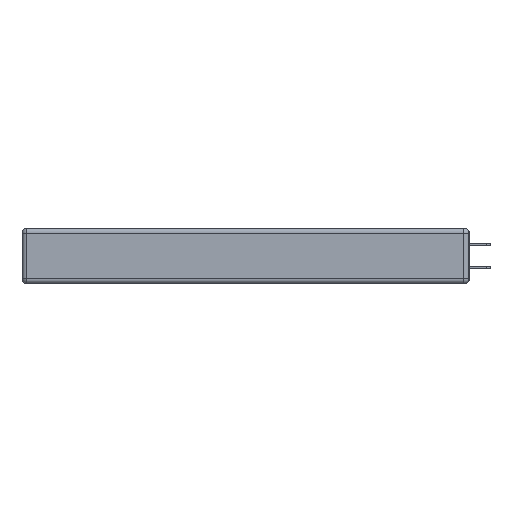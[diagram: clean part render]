
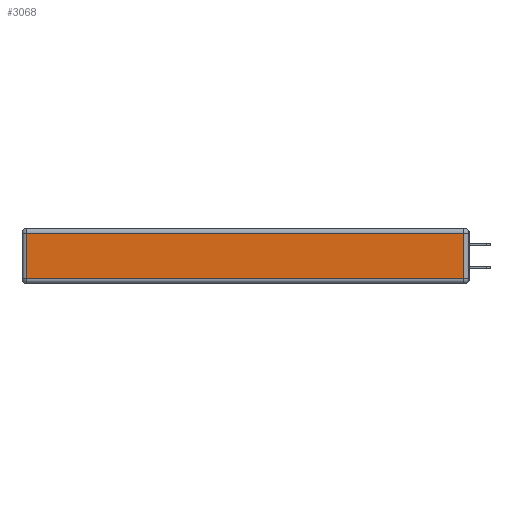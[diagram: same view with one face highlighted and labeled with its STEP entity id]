
A CAD part, left-side view. The second image highlights one B-rep face of the part: STEP entity #3068.
In plain terms, the highlighted planar face has unit normal (-1, 0, 0).
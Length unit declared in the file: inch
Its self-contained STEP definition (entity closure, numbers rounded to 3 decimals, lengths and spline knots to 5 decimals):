
#97 = CARTESIAN_POINT ( 'NONE',  ( 0., 2.72, -0.343 ) ) ;
#1035 = EDGE_CURVE ( 'NONE', #3423, #1359, #10766, .T. ) ;
#1359 = VERTEX_POINT ( 'NONE', #2898 ) ;
#1588 = CARTESIAN_POINT ( 'NONE',  ( 0., 0., -0.313 ) ) ;
#1816 = DIRECTION ( 'NONE',  ( 0., 0., 1. ) ) ;
#1874 = PLANE ( 'NONE',  #13687 ) ;
#2028 = ORIENTED_EDGE ( 'NONE', *, *, #1035, .T. ) ;
#2550 = FACE_OUTER_BOUND ( 'NONE', #21131, .T. ) ;
#2898 = CARTESIAN_POINT ( 'NONE',  ( 0., 0.03, -0.03 ) ) ;
#3068 = ADVANCED_FACE ( 'NONE', ( #2550 ), #1874, .T. ) ;
#3423 = VERTEX_POINT ( 'NONE', #15539 ) ;
#3523 = DIRECTION ( 'NONE',  ( 0., 0., -1. ) ) ;
#5363 = LINE ( 'NONE', #8226, #16827 ) ;
#6672 = ORIENTED_EDGE ( 'NONE', *, *, #12257, .T. ) ;
#6879 = DIRECTION ( 'NONE',  ( 0., -1., 0. ) ) ;
#7177 = ORIENTED_EDGE ( 'NONE', *, *, #19408, .T. ) ;
#8226 = CARTESIAN_POINT ( 'NONE',  ( 0., 2.75, -0.03 ) ) ;
#8332 = CARTESIAN_POINT ( 'NONE',  ( 0., 2.72, -0.03 ) ) ;
#9292 = EDGE_CURVE ( 'NONE', #10362, #3423, #16250, .T. ) ;
#9904 = CARTESIAN_POINT ( 'NONE',  ( 0., 2.72, -0.313 ) ) ;
#10362 = VERTEX_POINT ( 'NONE', #9904 ) ;
#10766 = LINE ( 'NONE', #20699, #14405 ) ;
#11316 = VECTOR ( 'NONE', #3523, 39.37008 ) ;
#11708 = DIRECTION ( 'NONE',  ( 0., 1., 0. ) ) ;
#12257 = EDGE_CURVE ( 'NONE', #20969, #10362, #16113, .T. ) ;
#12524 = DIRECTION ( 'NONE',  ( -1., 0., 0. ) ) ;
#13687 = AXIS2_PLACEMENT_3D ( 'NONE', #21454, #12524, #1816 ) ;
#14405 = VECTOR ( 'NONE', #22496, 39.37008 ) ;
#15539 = CARTESIAN_POINT ( 'NONE',  ( 0., 0.03, -0.313 ) ) ;
#16113 = LINE ( 'NONE', #97, #11316 ) ;
#16250 = LINE ( 'NONE', #1588, #20176 ) ;
#16827 = VECTOR ( 'NONE', #11708, 39.37008 ) ;
#19408 = EDGE_CURVE ( 'NONE', #1359, #20969, #5363, .T. ) ;
#20176 = VECTOR ( 'NONE', #6879, 39.37008 ) ;
#20401 = ORIENTED_EDGE ( 'NONE', *, *, #9292, .T. ) ;
#20699 = CARTESIAN_POINT ( 'NONE',  ( 0., 0.03, -0.343 ) ) ;
#20969 = VERTEX_POINT ( 'NONE', #8332 ) ;
#21131 = EDGE_LOOP ( 'NONE', ( #20401, #2028, #7177, #6672 ) ) ;
#21454 = CARTESIAN_POINT ( 'NONE',  ( 0., 0., -0.343 ) ) ;
#22496 = DIRECTION ( 'NONE',  ( 0., 0., 1. ) ) ;
